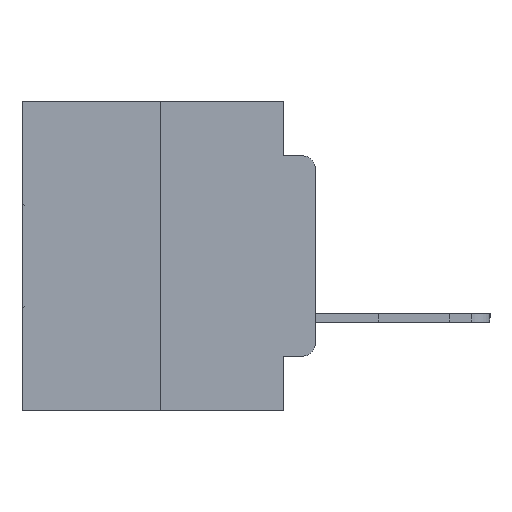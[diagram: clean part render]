
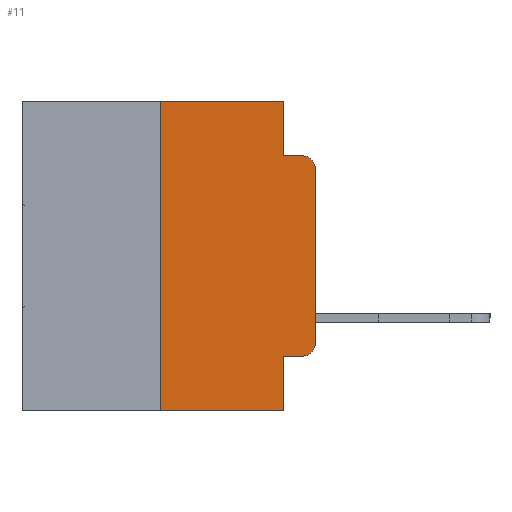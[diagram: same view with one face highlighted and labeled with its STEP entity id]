
A CAD part, left-side view. The second image highlights one B-rep face of the part: STEP entity #11.
In plain terms, the highlighted planar face has unit normal (-1, 0, 0).
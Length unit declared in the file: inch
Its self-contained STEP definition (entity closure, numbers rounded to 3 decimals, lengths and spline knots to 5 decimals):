
#11 = ADVANCED_FACE ( 'NONE', ( #8025 ), #3783, .F. ) ;
#323 = CARTESIAN_POINT ( 'NONE',  ( 0., 0., -0.1085 ) ) ;
#576 = CARTESIAN_POINT ( 'NONE',  ( 0., 0.02, -0.0885 ) ) ;
#1455 = LINE ( 'NONE', #1602, #7178 ) ;
#1565 = CARTESIAN_POINT ( 'NONE',  ( 0., 0.051, -0.5 ) ) ;
#1602 = CARTESIAN_POINT ( 'NONE',  ( 0., 0.051, -0.0885 ) ) ;
#1800 = VECTOR ( 'NONE', #26593, 39.37008 ) ;
#2025 = VECTOR ( 'NONE', #19343, 39.37008 ) ;
#2080 = ORIENTED_EDGE ( 'NONE', *, *, #24078, .F. ) ;
#2796 = LINE ( 'NONE', #9609, #2025 ) ;
#2929 = CARTESIAN_POINT ( 'NONE',  ( 0., 0.25, 0. ) ) ;
#3628 = ORIENTED_EDGE ( 'NONE', *, *, #8531, .F. ) ;
#3783 = PLANE ( 'NONE',  #28264 ) ;
#3968 = CARTESIAN_POINT ( 'NONE',  ( 0., 0., -0.3915 ) ) ;
#4065 = DIRECTION ( 'NONE',  ( 0., -1., 0. ) ) ;
#4430 = EDGE_CURVE ( 'NONE', #6587, #27908, #16424, .T. ) ;
#5550 = EDGE_CURVE ( 'NONE', #25482, #18664, #11780, .T. ) ;
#5716 = EDGE_CURVE ( 'NONE', #6568, #10797, #1455, .T. ) ;
#5775 = CARTESIAN_POINT ( 'NONE',  ( 0., 0.25, 0. ) ) ;
#5905 = ORIENTED_EDGE ( 'NONE', *, *, #4430, .T. ) ;
#6278 = ORIENTED_EDGE ( 'NONE', *, *, #29971, .T. ) ;
#6530 = CARTESIAN_POINT ( 'NONE',  ( 0., 0.02, -0.3915 ) ) ;
#6568 = VERTEX_POINT ( 'NONE', #30386 ) ;
#6587 = VERTEX_POINT ( 'NONE', #25820 ) ;
#6950 = DIRECTION ( 'NONE',  ( 0., 0., -1. ) ) ;
#7178 = VECTOR ( 'NONE', #4065, 39.37008 ) ;
#8025 = FACE_OUTER_BOUND ( 'NONE', #29363, .T. ) ;
#8183 = CARTESIAN_POINT ( 'NONE',  ( 0., 0.473, 0. ) ) ;
#8316 = CARTESIAN_POINT ( 'NONE',  ( 0., 0.051, 0. ) ) ;
#8362 = VECTOR ( 'NONE', #17846, 39.37008 ) ;
#8366 = VERTEX_POINT ( 'NONE', #323 ) ;
#8531 = EDGE_CURVE ( 'NONE', #25482, #16765, #18369, .T. ) ;
#8930 = DIRECTION ( 'NONE',  ( 0., 0., -1. ) ) ;
#9117 = CIRCLE ( 'NONE', #30485, 0.02 ) ;
#9609 = CARTESIAN_POINT ( 'NONE',  ( 0., 0.051, 0. ) ) ;
#10728 = VECTOR ( 'NONE', #11982, 39.37008 ) ;
#10797 = VERTEX_POINT ( 'NONE', #576 ) ;
#11195 = DIRECTION ( 'NONE',  ( 1., 0., 0. ) ) ;
#11465 = LINE ( 'NONE', #27326, #20434 ) ;
#11780 = LINE ( 'NONE', #22756, #24643 ) ;
#11982 = DIRECTION ( 'NONE',  ( 0., -1., 0. ) ) ;
#12797 = CARTESIAN_POINT ( 'NONE',  ( 0., 0.02, -0.1085 ) ) ;
#12941 = DIRECTION ( 'NONE',  ( 0., -1., 0. ) ) ;
#13067 = EDGE_CURVE ( 'NONE', #27908, #16670, #9117, .T. ) ;
#14637 = LINE ( 'NONE', #24235, #1800 ) ;
#15233 = DIRECTION ( 'NONE',  ( 0., 0., -1. ) ) ;
#15497 = CARTESIAN_POINT ( 'NONE',  ( 0., 0.051, 0. ) ) ;
#15968 = EDGE_CURVE ( 'NONE', #16765, #30084, #11465, .T. ) ;
#16130 = CARTESIAN_POINT ( 'NONE',  ( 0., 0.02, -0.4115 ) ) ;
#16424 = LINE ( 'NONE', #16979, #10728 ) ;
#16670 = VERTEX_POINT ( 'NONE', #3968 ) ;
#16765 = VERTEX_POINT ( 'NONE', #2929 ) ;
#16979 = CARTESIAN_POINT ( 'NONE',  ( 0., 0.051, -0.4115 ) ) ;
#17213 = ORIENTED_EDGE ( 'NONE', *, *, #22028, .F. ) ;
#17599 = VECTOR ( 'NONE', #27380, 39.37008 ) ;
#17846 = DIRECTION ( 'NONE',  ( 0., 0., -1. ) ) ;
#18004 = DIRECTION ( 'NONE',  ( 0., -1., 0. ) ) ;
#18354 = ORIENTED_EDGE ( 'NONE', *, *, #23122, .T. ) ;
#18369 = LINE ( 'NONE', #5775, #17599 ) ;
#18664 = VERTEX_POINT ( 'NONE', #1565 ) ;
#18745 = ORIENTED_EDGE ( 'NONE', *, *, #13067, .T. ) ;
#19343 = DIRECTION ( 'NONE',  ( 0., 0., -1. ) ) ;
#20434 = VECTOR ( 'NONE', #12941, 39.37008 ) ;
#21166 = LINE ( 'NONE', #15497, #8362 ) ;
#21349 = ORIENTED_EDGE ( 'NONE', *, *, #15968, .F. ) ;
#22028 = EDGE_CURVE ( 'NONE', #6587, #18664, #21166, .T. ) ;
#22064 = AXIS2_PLACEMENT_3D ( 'NONE', #12797, #29511, #15233 ) ;
#22756 = CARTESIAN_POINT ( 'NONE',  ( 0., 0.473, -0.5 ) ) ;
#23122 = EDGE_CURVE ( 'NONE', #16670, #8366, #14637, .T. ) ;
#23387 = DIRECTION ( 'NONE',  ( -1., 0., 0. ) ) ;
#24078 = EDGE_CURVE ( 'NONE', #30084, #6568, #2796, .T. ) ;
#24235 = CARTESIAN_POINT ( 'NONE',  ( 0., 0., 0. ) ) ;
#24643 = VECTOR ( 'NONE', #18004, 39.37008 ) ;
#25480 = ORIENTED_EDGE ( 'NONE', *, *, #5716, .F. ) ;
#25482 = VERTEX_POINT ( 'NONE', #30617 ) ;
#25820 = CARTESIAN_POINT ( 'NONE',  ( 0., 0.051, -0.4115 ) ) ;
#26593 = DIRECTION ( 'NONE',  ( 0., 0., 1. ) ) ;
#27246 = CIRCLE ( 'NONE', #22064, 0.02 ) ;
#27326 = CARTESIAN_POINT ( 'NONE',  ( 0., 0.473, 0. ) ) ;
#27380 = DIRECTION ( 'NONE',  ( 0., 0., 1. ) ) ;
#27908 = VERTEX_POINT ( 'NONE', #16130 ) ;
#28264 = AXIS2_PLACEMENT_3D ( 'NONE', #8183, #11195, #6950 ) ;
#29099 = ORIENTED_EDGE ( 'NONE', *, *, #5550, .T. ) ;
#29363 = EDGE_LOOP ( 'NONE', ( #18354, #6278, #25480, #2080, #21349, #3628, #29099, #17213, #5905, #18745 ) ) ;
#29511 = DIRECTION ( 'NONE',  ( -1., 0., 0. ) ) ;
#29971 = EDGE_CURVE ( 'NONE', #8366, #10797, #27246, .T. ) ;
#30084 = VERTEX_POINT ( 'NONE', #8316 ) ;
#30386 = CARTESIAN_POINT ( 'NONE',  ( 0., 0.051, -0.0885 ) ) ;
#30485 = AXIS2_PLACEMENT_3D ( 'NONE', #6530, #23387, #8930 ) ;
#30617 = CARTESIAN_POINT ( 'NONE',  ( 0., 0.25, -0.5 ) ) ;
